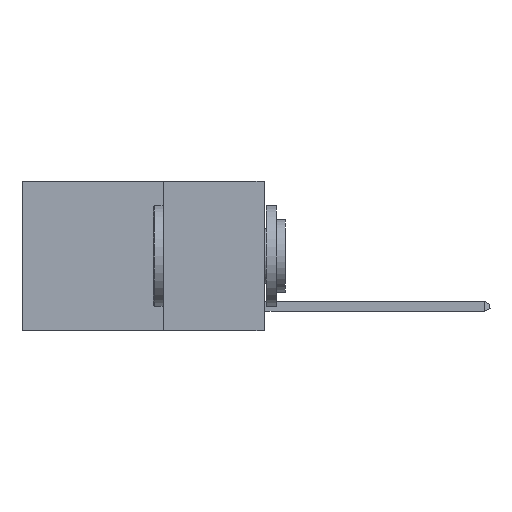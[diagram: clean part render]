
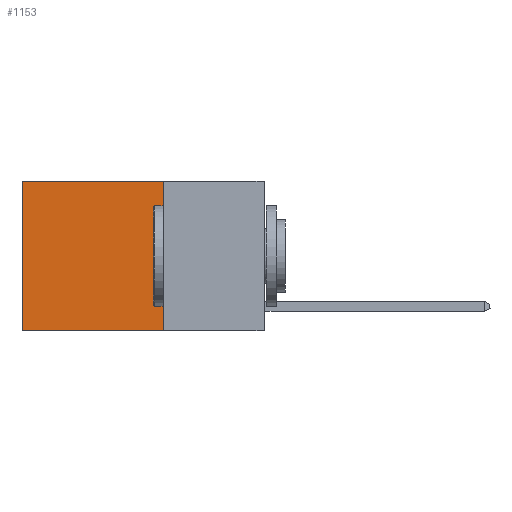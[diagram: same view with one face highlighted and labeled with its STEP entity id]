
A CAD part, left-side view. The second image highlights one B-rep face of the part: STEP entity #1153.
In plain terms, the highlighted planar face has unit normal (-1, 0, 0).
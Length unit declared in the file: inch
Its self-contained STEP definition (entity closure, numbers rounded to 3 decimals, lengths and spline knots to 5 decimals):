
#848 = CARTESIAN_POINT ( 'NONE',  ( 0.2625, 0.25, 0. ) ) ;
#960 = AXIS2_PLACEMENT_3D ( 'NONE', #1304, #5717, #1094 ) ;
#1008 = CARTESIAN_POINT ( 'NONE',  ( 0.2625, 0.25, 0. ) ) ;
#1094 = DIRECTION ( 'NONE',  ( 0., 0., -1. ) ) ;
#1153 = ADVANCED_FACE ( 'NONE', ( #3511 ), #12332, .F. ) ;
#1304 = CARTESIAN_POINT ( 'NONE',  ( 0.2625, 0.25, 0. ) ) ;
#1695 = LINE ( 'NONE', #4954, #4076 ) ;
#1798 = VERTEX_POINT ( 'NONE', #13984 ) ;
#2276 = VECTOR ( 'NONE', #7107, 39.37008 ) ;
#2503 = CARTESIAN_POINT ( 'NONE',  ( 0.2625, 0.25, 0. ) ) ;
#2892 = VERTEX_POINT ( 'NONE', #1008 ) ;
#3169 = CARTESIAN_POINT ( 'NONE',  ( 0.2625, 0.25, -0.37 ) ) ;
#3255 = CARTESIAN_POINT ( 'NONE',  ( 0.2625, 0.6, 0. ) ) ;
#3511 = FACE_OUTER_BOUND ( 'NONE', #4312, .T. ) ;
#3654 = EDGE_CURVE ( 'NONE', #2892, #9538, #4298, .T. ) ;
#3996 = EDGE_CURVE ( 'NONE', #9538, #1798, #1695, .T. ) ;
#4076 = VECTOR ( 'NONE', #9368, 39.37008 ) ;
#4298 = LINE ( 'NONE', #848, #12285 ) ;
#4312 = EDGE_LOOP ( 'NONE', ( #14202, #10900, #14031, #4406 ) ) ;
#4406 = ORIENTED_EDGE ( 'NONE', *, *, #7731, .T. ) ;
#4954 = CARTESIAN_POINT ( 'NONE',  ( 0.2625, 0.25, -0.37 ) ) ;
#5041 = VERTEX_POINT ( 'NONE', #5327 ) ;
#5325 = DIRECTION ( 'NONE',  ( 0., 0., -1. ) ) ;
#5327 = CARTESIAN_POINT ( 'NONE',  ( 0.2625, 0.6, 0. ) ) ;
#5717 = DIRECTION ( 'NONE',  ( 1., 0., 0. ) ) ;
#5902 = LINE ( 'NONE', #2503, #2276 ) ;
#6697 = EDGE_CURVE ( 'NONE', #5041, #1798, #13330, .T. ) ;
#7107 = DIRECTION ( 'NONE',  ( 0., 1., 0. ) ) ;
#7599 = DIRECTION ( 'NONE',  ( 0., 0., -1. ) ) ;
#7731 = EDGE_CURVE ( 'NONE', #2892, #5041, #5902, .T. ) ;
#9368 = DIRECTION ( 'NONE',  ( 0., 1., 0. ) ) ;
#9538 = VERTEX_POINT ( 'NONE', #3169 ) ;
#10900 = ORIENTED_EDGE ( 'NONE', *, *, #3996, .F. ) ;
#12285 = VECTOR ( 'NONE', #5325, 39.37008 ) ;
#12332 = PLANE ( 'NONE',  #960 ) ;
#13330 = LINE ( 'NONE', #3255, #14037 ) ;
#13984 = CARTESIAN_POINT ( 'NONE',  ( 0.2625, 0.6, -0.37 ) ) ;
#14031 = ORIENTED_EDGE ( 'NONE', *, *, #3654, .F. ) ;
#14037 = VECTOR ( 'NONE', #7599, 39.37008 ) ;
#14202 = ORIENTED_EDGE ( 'NONE', *, *, #6697, .T. ) ;
